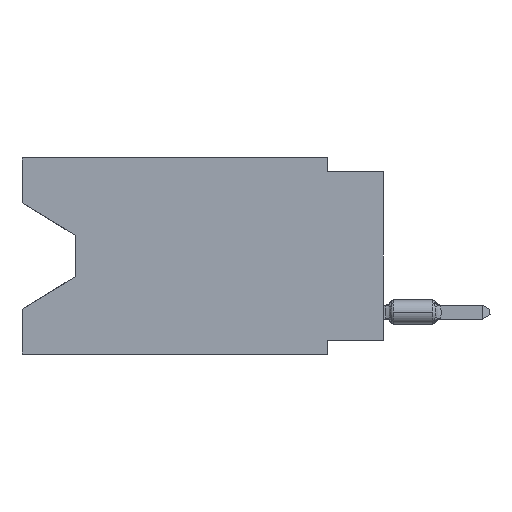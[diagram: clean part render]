
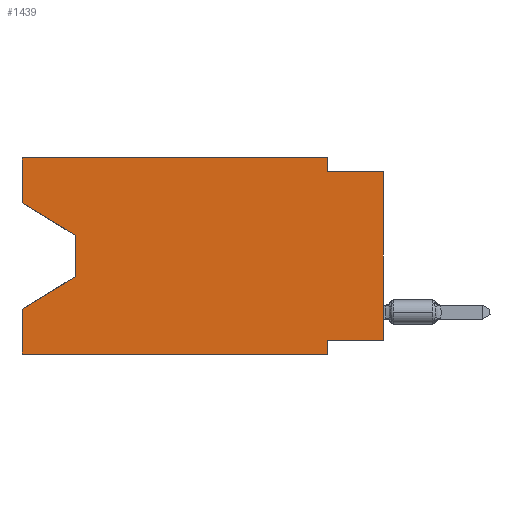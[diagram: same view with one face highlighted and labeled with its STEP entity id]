
A CAD part, left-side view. The second image highlights one B-rep face of the part: STEP entity #1439.
In plain terms, the highlighted planar face has unit normal (-1, 0, 0).
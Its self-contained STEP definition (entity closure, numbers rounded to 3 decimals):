
#1310 = ORIENTED_EDGE ( 'NONE', *, *, #5079, .F. ) ;
#1439 = ADVANCED_FACE ( 'NONE', ( #2611 ), #22088, .F. ) ;
#1888 = CARTESIAN_POINT ( 'NONE',  ( 0., 2.54, -8.89 ) ) ;
#2611 = FACE_OUTER_BOUND ( 'NONE', #14281, .T. ) ;
#2795 = ORIENTED_EDGE ( 'NONE', *, *, #41404, .T. ) ;
#4133 = LINE ( 'NONE', #22701, #56153 ) ;
#4570 = VERTEX_POINT ( 'NONE', #30098 ) ;
#5079 = EDGE_CURVE ( 'NONE', #16263, #22809, #4133, .T. ) ;
#5842 = ORIENTED_EDGE ( 'NONE', *, *, #39448, .F. ) ;
#8338 = CARTESIAN_POINT ( 'NONE',  ( 0., 2.54, 0. ) ) ;
#8803 = CARTESIAN_POINT ( 'NONE',  ( 0., 16.383, -8.89 ) ) ;
#9447 = EDGE_CURVE ( 'NONE', #46821, #37859, #23055, .T. ) ;
#9686 = ORIENTED_EDGE ( 'NONE', *, *, #42270, .F. ) ;
#10940 = CARTESIAN_POINT ( 'NONE',  ( 0., 16.383, 0. ) ) ;
#11229 = LINE ( 'NONE', #54202, #23424 ) ;
#11398 = ORIENTED_EDGE ( 'NONE', *, *, #22483, .T. ) ;
#12581 = VERTEX_POINT ( 'NONE', #56120 ) ;
#13162 = CARTESIAN_POINT ( 'NONE',  ( 0., 16.383, 0. ) ) ;
#13253 = DIRECTION ( 'NONE',  ( 0., 0.855, -0.519 ) ) ;
#13610 = CARTESIAN_POINT ( 'NONE',  ( 0., 2.54, 0. ) ) ;
#13923 = ORIENTED_EDGE ( 'NONE', *, *, #27162, .F. ) ;
#14281 = EDGE_LOOP ( 'NONE', ( #2795, #41742, #26690, #15362, #11398, #9686, #1310, #15039, #5842, #36887, #39629, #13923 ) ) ;
#14328 = LINE ( 'NONE', #50960, #51132 ) ;
#15039 = ORIENTED_EDGE ( 'NONE', *, *, #17866, .T. ) ;
#15362 = ORIENTED_EDGE ( 'NONE', *, *, #42674, .F. ) ;
#16263 = VERTEX_POINT ( 'NONE', #29026 ) ;
#16904 = CARTESIAN_POINT ( 'NONE',  ( 0., 16.383, 0. ) ) ;
#17685 = VECTOR ( 'NONE', #36652, 1000. ) ;
#17866 = EDGE_CURVE ( 'NONE', #16263, #44377, #58901, .T. ) ;
#20006 = CARTESIAN_POINT ( 'NONE',  ( 0., 2.54, -8.255 ) ) ;
#21353 = VERTEX_POINT ( 'NONE', #22492 ) ;
#22088 = PLANE ( 'NONE',  #33619 ) ;
#22483 = EDGE_CURVE ( 'NONE', #4570, #21353, #54530, .T. ) ;
#22492 = CARTESIAN_POINT ( 'NONE',  ( 0., 2.54, -8.89 ) ) ;
#22701 = CARTESIAN_POINT ( 'NONE',  ( 0., 0., -8.255 ) ) ;
#22809 = VERTEX_POINT ( 'NONE', #20006 ) ;
#23055 = LINE ( 'NONE', #13610, #43964 ) ;
#23424 = VECTOR ( 'NONE', #29529, 1000. ) ;
#26690 = ORIENTED_EDGE ( 'NONE', *, *, #45587, .T. ) ;
#27162 = EDGE_CURVE ( 'NONE', #56602, #38094, #11229, .T. ) ;
#27978 = VERTEX_POINT ( 'NONE', #58052 ) ;
#29026 = CARTESIAN_POINT ( 'NONE',  ( 0., 0., -8.255 ) ) ;
#29529 = DIRECTION ( 'NONE',  ( 0., 0., 1. ) ) ;
#30098 = CARTESIAN_POINT ( 'NONE',  ( 0., 16.383, -8.89 ) ) ;
#30583 = VECTOR ( 'NONE', #53842, 1000. ) ;
#31216 = DIRECTION ( 'NONE',  ( 0., -1., 0. ) ) ;
#31525 = CARTESIAN_POINT ( 'NONE',  ( 0., 0., -0.635 ) ) ;
#32371 = LINE ( 'NONE', #13162, #17685 ) ;
#33619 = AXIS2_PLACEMENT_3D ( 'NONE', #16904, #54734, #59014 ) ;
#33874 = VERTEX_POINT ( 'NONE', #56313 ) ;
#36652 = DIRECTION ( 'NONE',  ( 0., -1., 0. ) ) ;
#36887 = ORIENTED_EDGE ( 'NONE', *, *, #9447, .F. ) ;
#37098 = DIRECTION ( 'NONE',  ( 0., 0., -1. ) ) ;
#37322 = VECTOR ( 'NONE', #39291, 1000. ) ;
#37859 = VERTEX_POINT ( 'NONE', #47263 ) ;
#38094 = VERTEX_POINT ( 'NONE', #47413 ) ;
#38767 = DIRECTION ( 'NONE',  ( 0., 0., -1. ) ) ;
#38904 = EDGE_CURVE ( 'NONE', #38094, #46821, #32371, .T. ) ;
#39291 = DIRECTION ( 'NONE',  ( 0., 0., 1. ) ) ;
#39448 = EDGE_CURVE ( 'NONE', #37859, #44377, #54698, .T. ) ;
#39629 = ORIENTED_EDGE ( 'NONE', *, *, #38904, .F. ) ;
#40163 = VECTOR ( 'NONE', #31216, 1000. ) ;
#40579 = CARTESIAN_POINT ( 'NONE',  ( 0., 0., 0. ) ) ;
#41404 = EDGE_CURVE ( 'NONE', #56602, #33874, #49563, .T. ) ;
#41600 = CARTESIAN_POINT ( 'NONE',  ( 0., 13.97, -5.385 ) ) ;
#41742 = ORIENTED_EDGE ( 'NONE', *, *, #50694, .T. ) ;
#42270 = EDGE_CURVE ( 'NONE', #22809, #21353, #57670, .T. ) ;
#42653 = CARTESIAN_POINT ( 'NONE',  ( 0., 16.383, -2.038 ) ) ;
#42674 = EDGE_CURVE ( 'NONE', #4570, #12581, #53314, .T. ) ;
#43964 = VECTOR ( 'NONE', #37098, 1000. ) ;
#44377 = VERTEX_POINT ( 'NONE', #54706 ) ;
#45587 = EDGE_CURVE ( 'NONE', #27978, #12581, #55047, .T. ) ;
#46821 = VERTEX_POINT ( 'NONE', #8338 ) ;
#47263 = CARTESIAN_POINT ( 'NONE',  ( 0., 2.54, -0.635 ) ) ;
#47413 = CARTESIAN_POINT ( 'NONE',  ( 0., 16.383, 0. ) ) ;
#49124 = DIRECTION ( 'NONE',  ( 0., 0., 1. ) ) ;
#49258 = CARTESIAN_POINT ( 'NONE',  ( 0., 16.383, -2.038 ) ) ;
#49563 = LINE ( 'NONE', #49258, #30583 ) ;
#50694 = EDGE_CURVE ( 'NONE', #33874, #27978, #14328, .T. ) ;
#50960 = CARTESIAN_POINT ( 'NONE',  ( 0., 13.97, -3.505 ) ) ;
#51132 = VECTOR ( 'NONE', #51849, 1000. ) ;
#51849 = DIRECTION ( 'NONE',  ( 0., 0., -1. ) ) ;
#52414 = VECTOR ( 'NONE', #49124, 1000. ) ;
#53314 = LINE ( 'NONE', #10940, #37322 ) ;
#53842 = DIRECTION ( 'NONE',  ( 0., -0.855, -0.519 ) ) ;
#54202 = CARTESIAN_POINT ( 'NONE',  ( 0., 16.383, 0. ) ) ;
#54530 = LINE ( 'NONE', #8803, #59834 ) ;
#54698 = LINE ( 'NONE', #31525, #40163 ) ;
#54706 = CARTESIAN_POINT ( 'NONE',  ( 0., 0., -0.635 ) ) ;
#54734 = DIRECTION ( 'NONE',  ( 1., 0., 0. ) ) ;
#55047 = LINE ( 'NONE', #41600, #59120 ) ;
#55340 = DIRECTION ( 'NONE',  ( 0., 1., 0. ) ) ;
#56120 = CARTESIAN_POINT ( 'NONE',  ( 0., 16.383, -6.852 ) ) ;
#56153 = VECTOR ( 'NONE', #55340, 1000. ) ;
#56313 = CARTESIAN_POINT ( 'NONE',  ( 0., 13.97, -3.505 ) ) ;
#56602 = VERTEX_POINT ( 'NONE', #42653 ) ;
#57670 = LINE ( 'NONE', #1888, #59749 ) ;
#58052 = CARTESIAN_POINT ( 'NONE',  ( 0., 13.97, -5.385 ) ) ;
#58811 = DIRECTION ( 'NONE',  ( 0., -1., 0. ) ) ;
#58901 = LINE ( 'NONE', #40579, #52414 ) ;
#59014 = DIRECTION ( 'NONE',  ( 0., 0., -1. ) ) ;
#59120 = VECTOR ( 'NONE', #13253, 1000. ) ;
#59749 = VECTOR ( 'NONE', #38767, 1000. ) ;
#59834 = VECTOR ( 'NONE', #58811, 1000. ) ;
